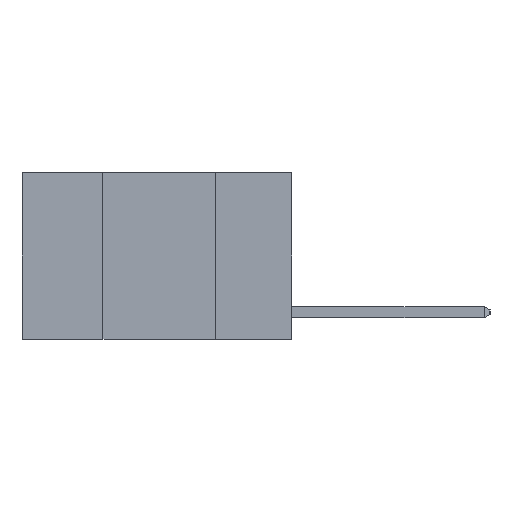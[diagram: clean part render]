
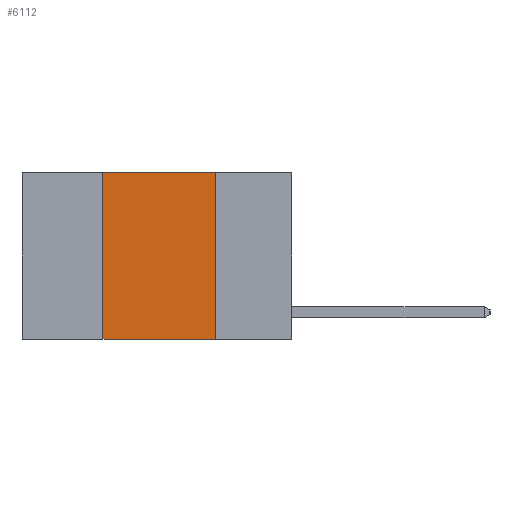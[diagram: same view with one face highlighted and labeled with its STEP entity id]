
A CAD part, left-side view. The second image highlights one B-rep face of the part: STEP entity #6112.
In plain terms, the highlighted planar face has unit normal (-1, 0, 0).
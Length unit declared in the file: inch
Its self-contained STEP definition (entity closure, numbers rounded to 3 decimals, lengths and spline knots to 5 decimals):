
#82 = CARTESIAN_POINT ( 'NONE',  ( 0., 0.42, 0. ) ) ;
#107 = LINE ( 'NONE', #8341, #1815 ) ;
#429 = PLANE ( 'NONE',  #5954 ) ;
#430 = FACE_OUTER_BOUND ( 'NONE', #2877, .T. ) ;
#806 = VERTEX_POINT ( 'NONE', #7149 ) ;
#909 = ORIENTED_EDGE ( 'NONE', *, *, #7743, .F. ) ;
#982 = LINE ( 'NONE', #4614, #8269 ) ;
#1171 = DIRECTION ( 'NONE',  ( 1., 0., 0. ) ) ;
#1815 = VECTOR ( 'NONE', #3733, 39.37008 ) ;
#2215 = VERTEX_POINT ( 'NONE', #82 ) ;
#2446 = ORIENTED_EDGE ( 'NONE', *, *, #8280, .F. ) ;
#2532 = CARTESIAN_POINT ( 'NONE',  ( 0., 0.6, 0. ) ) ;
#2877 = EDGE_LOOP ( 'NONE', ( #2446, #909, #2882, #6664 ) ) ;
#2882 = ORIENTED_EDGE ( 'NONE', *, *, #4077, .F. ) ;
#3216 = CARTESIAN_POINT ( 'NONE',  ( 0., 0.17, -0.37 ) ) ;
#3733 = DIRECTION ( 'NONE',  ( 0., 0., 1. ) ) ;
#4077 = EDGE_CURVE ( 'NONE', #7083, #2215, #107, .T. ) ;
#4102 = CARTESIAN_POINT ( 'NONE',  ( 0., 0.17, 0. ) ) ;
#4309 = CARTESIAN_POINT ( 'NONE',  ( 0., 0.6, 0. ) ) ;
#4614 = CARTESIAN_POINT ( 'NONE',  ( 0., 0.6, -0.37 ) ) ;
#4772 = DIRECTION ( 'NONE',  ( 0., 0., -1. ) ) ;
#5261 = DIRECTION ( 'NONE',  ( 0., -1., 0. ) ) ;
#5498 = LINE ( 'NONE', #4309, #8564 ) ;
#5831 = DIRECTION ( 'NONE',  ( 0., 0., -1. ) ) ;
#5954 = AXIS2_PLACEMENT_3D ( 'NONE', #2532, #1171, #5831 ) ;
#6112 = ADVANCED_FACE ( 'NONE', ( #430 ), #429, .F. ) ;
#6394 = VECTOR ( 'NONE', #4772, 39.37008 ) ;
#6664 = ORIENTED_EDGE ( 'NONE', *, *, #8093, .T. ) ;
#7083 = VERTEX_POINT ( 'NONE', #8270 ) ;
#7149 = CARTESIAN_POINT ( 'NONE',  ( 0., 0.17, 0. ) ) ;
#7565 = DIRECTION ( 'NONE',  ( 0., -1., 0. ) ) ;
#7743 = EDGE_CURVE ( 'NONE', #2215, #806, #5498, .T. ) ;
#8069 = VERTEX_POINT ( 'NONE', #3216 ) ;
#8093 = EDGE_CURVE ( 'NONE', #7083, #8069, #982, .T. ) ;
#8165 = LINE ( 'NONE', #4102, #6394 ) ;
#8269 = VECTOR ( 'NONE', #5261, 39.37008 ) ;
#8270 = CARTESIAN_POINT ( 'NONE',  ( 0., 0.42, -0.37 ) ) ;
#8280 = EDGE_CURVE ( 'NONE', #806, #8069, #8165, .T. ) ;
#8341 = CARTESIAN_POINT ( 'NONE',  ( 0., 0.42, 0. ) ) ;
#8564 = VECTOR ( 'NONE', #7565, 39.37008 ) ;
